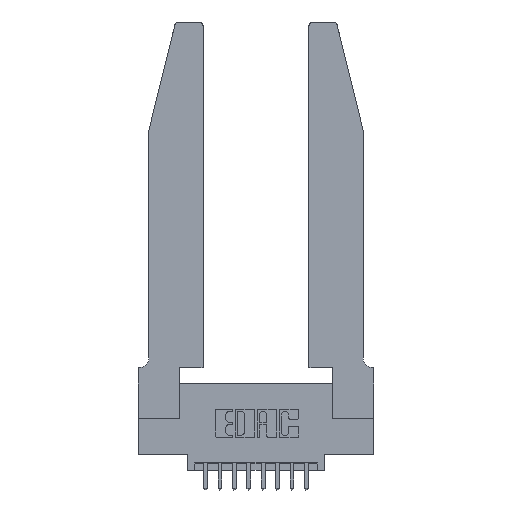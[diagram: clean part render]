
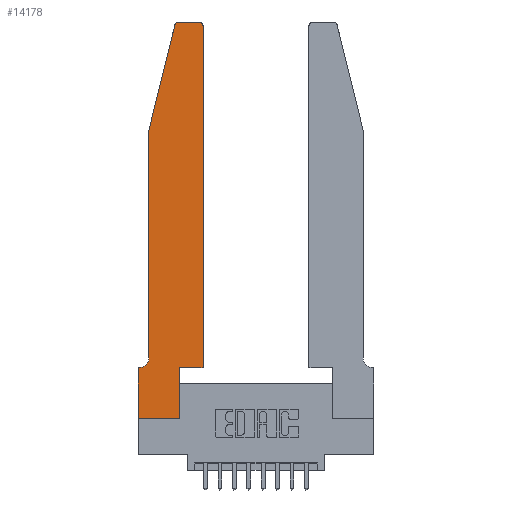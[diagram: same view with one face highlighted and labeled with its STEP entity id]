
A CAD part, top view. The second image highlights one B-rep face of the part: STEP entity #14178.
In plain terms, the highlighted planar face has unit normal (0, 0, 1).
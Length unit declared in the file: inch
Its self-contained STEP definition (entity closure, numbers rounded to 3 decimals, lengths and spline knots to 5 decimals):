
#3 = ORIENTED_EDGE ( 'NONE', *, *, #5869, .T. ) ;
#110 = LINE ( 'NONE', #14669, #13634 ) ;
#135 = ORIENTED_EDGE ( 'NONE', *, *, #9472, .T. ) ;
#204 = DIRECTION ( 'NONE',  ( -1., 0., 0. ) ) ;
#494 = LINE ( 'NONE', #12184, #2586 ) ;
#677 = CARTESIAN_POINT ( 'NONE',  ( 0.4505, 2.72, 0.37 ) ) ;
#746 = DIRECTION ( 'NONE',  ( 0., -1., 0. ) ) ;
#749 = VERTEX_POINT ( 'NONE', #677 ) ;
#1006 = VECTOR ( 'NONE', #10287, 39.37008 ) ;
#1123 = CARTESIAN_POINT ( 'NONE',  ( 0., 0.35, 0.37 ) ) ;
#1142 = CARTESIAN_POINT ( 'NONE',  ( 0.25487, 2.72718, 0.37 ) ) ;
#1192 = CARTESIAN_POINT ( 'NONE',  ( 0.0755, 2., 0.37 ) ) ;
#1410 = AXIS2_PLACEMENT_3D ( 'NONE', #2428, #10925, #204 ) ;
#1765 = DIRECTION ( 'NONE',  ( 0., 0., 1. ) ) ;
#2149 = CARTESIAN_POINT ( 'NONE',  ( 0.0755, 0.35, 0.37 ) ) ;
#2259 = CARTESIAN_POINT ( 'NONE',  ( 0.0755, 0.42, 0.37 ) ) ;
#2366 = LINE ( 'NONE', #4662, #14963 ) ;
#2428 = CARTESIAN_POINT ( 'NONE',  ( 0.0055, 0.42, 0.37 ) ) ;
#2586 = VECTOR ( 'NONE', #12342, 39.37008 ) ;
#2697 = CIRCLE ( 'NONE', #10093, 0.03 ) ;
#2794 = ORIENTED_EDGE ( 'NONE', *, *, #4607, .T. ) ;
#3088 = DIRECTION ( 'NONE',  ( 1., 0., 0. ) ) ;
#3093 = EDGE_CURVE ( 'NONE', #9676, #9361, #14293, .T. ) ;
#3122 = EDGE_CURVE ( 'NONE', #6740, #3856, #12200, .T. ) ;
#3150 = ORIENTED_EDGE ( 'NONE', *, *, #11182, .T. ) ;
#3248 = CARTESIAN_POINT ( 'NONE',  ( 0.2865, 0.35, 0.37 ) ) ;
#3325 = LINE ( 'NONE', #5766, #4843 ) ;
#3831 = VERTEX_POINT ( 'NONE', #11753 ) ;
#3856 = VERTEX_POINT ( 'NONE', #1142 ) ;
#4101 = VERTEX_POINT ( 'NONE', #5190 ) ;
#4607 = EDGE_CURVE ( 'NONE', #4101, #6168, #9406, .T. ) ;
#4662 = CARTESIAN_POINT ( 'NONE',  ( 0.0755, 2., 0.37 ) ) ;
#4683 = DIRECTION ( 'NONE',  ( -1., 0., 0. ) ) ;
#4740 = PLANE ( 'NONE',  #6748 ) ;
#4843 = VECTOR ( 'NONE', #11882, 39.37008 ) ;
#4899 = VERTEX_POINT ( 'NONE', #4945 ) ;
#4945 = CARTESIAN_POINT ( 'NONE',  ( 0.0055, 0.35, 0.37 ) ) ;
#5026 = EDGE_CURVE ( 'NONE', #3856, #13792, #2366, .T. ) ;
#5085 = EDGE_LOOP ( 'NONE', ( #9479, #5961, #11658, #135, #9441, #15532, #5302, #3150, #2794, #11672, #5651, #3 ) ) ;
#5190 = CARTESIAN_POINT ( 'NONE',  ( 0.2865, 0., 0.37 ) ) ;
#5285 = CARTESIAN_POINT ( 'NONE',  ( 0.0755, 2., 0.37 ) ) ;
#5302 = ORIENTED_EDGE ( 'NONE', *, *, #3093, .T. ) ;
#5405 = EDGE_CURVE ( 'NONE', #6168, #11157, #15512, .T. ) ;
#5462 = CARTESIAN_POINT ( 'NONE',  ( 0.4205, 2.72, 0.37 ) ) ;
#5651 = ORIENTED_EDGE ( 'NONE', *, *, #11567, .T. ) ;
#5660 = VECTOR ( 'NONE', #746, 39.37008 ) ;
#5766 = CARTESIAN_POINT ( 'NONE',  ( 0., 0., 0.37 ) ) ;
#5869 = EDGE_CURVE ( 'NONE', #749, #3831, #2697, .T. ) ;
#5961 = ORIENTED_EDGE ( 'NONE', *, *, #3122, .T. ) ;
#6168 = VERTEX_POINT ( 'NONE', #3248 ) ;
#6740 = VERTEX_POINT ( 'NONE', #9810 ) ;
#6748 = AXIS2_PLACEMENT_3D ( 'NONE', #1123, #13284, #7177 ) ;
#6801 = CIRCLE ( 'NONE', #1410, 0.07 ) ;
#7133 = CARTESIAN_POINT ( 'NONE',  ( 0.2865, 0.35, 0.37 ) ) ;
#7177 = DIRECTION ( 'NONE',  ( 1., 0., 0. ) ) ;
#7190 = CARTESIAN_POINT ( 'NONE',  ( 0., 0.35, 0.37 ) ) ;
#7384 = EDGE_CURVE ( 'NONE', #4899, #9676, #15258, .T. ) ;
#7447 = VERTEX_POINT ( 'NONE', #2259 ) ;
#8029 = EDGE_CURVE ( 'NONE', #7447, #4899, #6801, .T. ) ;
#9361 = VERTEX_POINT ( 'NONE', #11300 ) ;
#9406 = LINE ( 'NONE', #7133, #13404 ) ;
#9441 = ORIENTED_EDGE ( 'NONE', *, *, #8029, .T. ) ;
#9472 = EDGE_CURVE ( 'NONE', #13792, #7447, #9675, .T. ) ;
#9479 = ORIENTED_EDGE ( 'NONE', *, *, #10790, .T. ) ;
#9621 = DIRECTION ( 'NONE',  ( 0., 1., 0. ) ) ;
#9675 = LINE ( 'NONE', #5285, #13509 ) ;
#9676 = VERTEX_POINT ( 'NONE', #7190 ) ;
#9810 = CARTESIAN_POINT ( 'NONE',  ( 0.284, 2.75, 0.37 ) ) ;
#10093 = AXIS2_PLACEMENT_3D ( 'NONE', #5462, #14035, #3088 ) ;
#10199 = DIRECTION ( 'NONE',  ( 0., -1., 0. ) ) ;
#10287 = DIRECTION ( 'NONE',  ( 1., 0., 0. ) ) ;
#10289 = VECTOR ( 'NONE', #4683, 39.37008 ) ;
#10447 = CARTESIAN_POINT ( 'NONE',  ( 0.4505, 0.35, 0.37 ) ) ;
#10790 = EDGE_CURVE ( 'NONE', #3831, #6740, #494, .T. ) ;
#10886 = FACE_OUTER_BOUND ( 'NONE', #5085, .T. ) ;
#10925 = DIRECTION ( 'NONE',  ( 0., 0., -1. ) ) ;
#11157 = VERTEX_POINT ( 'NONE', #10447 ) ;
#11182 = EDGE_CURVE ( 'NONE', #9361, #4101, #3325, .T. ) ;
#11300 = CARTESIAN_POINT ( 'NONE',  ( 0., 0., 0.37 ) ) ;
#11567 = EDGE_CURVE ( 'NONE', #11157, #749, #110, .T. ) ;
#11658 = ORIENTED_EDGE ( 'NONE', *, *, #5026, .T. ) ;
#11672 = ORIENTED_EDGE ( 'NONE', *, *, #5405, .T. ) ;
#11753 = CARTESIAN_POINT ( 'NONE',  ( 0.4205, 2.75, 0.37 ) ) ;
#11882 = DIRECTION ( 'NONE',  ( 1., 0., 0. ) ) ;
#12184 = CARTESIAN_POINT ( 'NONE',  ( 0.2605, 2.75, 0.37 ) ) ;
#12200 = CIRCLE ( 'NONE', #15380, 0.03 ) ;
#12326 = DIRECTION ( 'NONE',  ( 0., 1., 0. ) ) ;
#12342 = DIRECTION ( 'NONE',  ( -1., 0., 0. ) ) ;
#13224 = DIRECTION ( 'NONE',  ( -0.239, -0.971, 0. ) ) ;
#13284 = DIRECTION ( 'NONE',  ( 0., 0., 1. ) ) ;
#13404 = VECTOR ( 'NONE', #9621, 39.37008 ) ;
#13489 = DIRECTION ( 'NONE',  ( 1., 0., 0. ) ) ;
#13509 = VECTOR ( 'NONE', #10199, 39.37008 ) ;
#13634 = VECTOR ( 'NONE', #12326, 39.37008 ) ;
#13792 = VERTEX_POINT ( 'NONE', #1192 ) ;
#14035 = DIRECTION ( 'NONE',  ( 0., 0., 1. ) ) ;
#14154 = CARTESIAN_POINT ( 'NONE',  ( 0., 0., 0.37 ) ) ;
#14178 = ADVANCED_FACE ( 'NONE', ( #10886 ), #4740, .T. ) ;
#14293 = LINE ( 'NONE', #14154, #5660 ) ;
#14669 = CARTESIAN_POINT ( 'NONE',  ( 0.4505, 0.35, 0.37 ) ) ;
#14963 = VECTOR ( 'NONE', #13224, 39.37008 ) ;
#15083 = CARTESIAN_POINT ( 'NONE',  ( 0.284, 2.72, 0.37 ) ) ;
#15195 = CARTESIAN_POINT ( 'NONE',  ( 0.4505, 0.35, 0.37 ) ) ;
#15258 = LINE ( 'NONE', #2149, #10289 ) ;
#15380 = AXIS2_PLACEMENT_3D ( 'NONE', #15083, #1765, #13489 ) ;
#15512 = LINE ( 'NONE', #15195, #1006 ) ;
#15532 = ORIENTED_EDGE ( 'NONE', *, *, #7384, .T. ) ;
